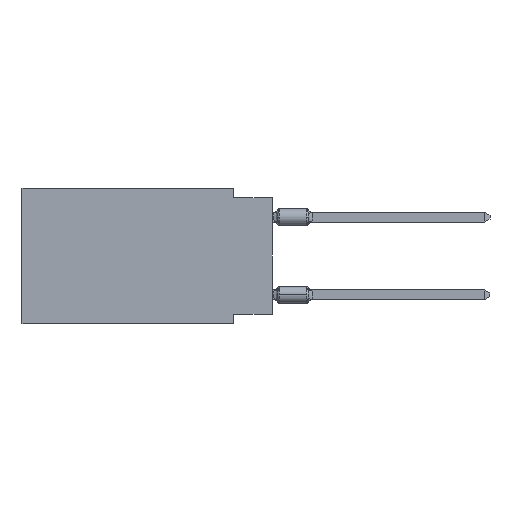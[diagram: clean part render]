
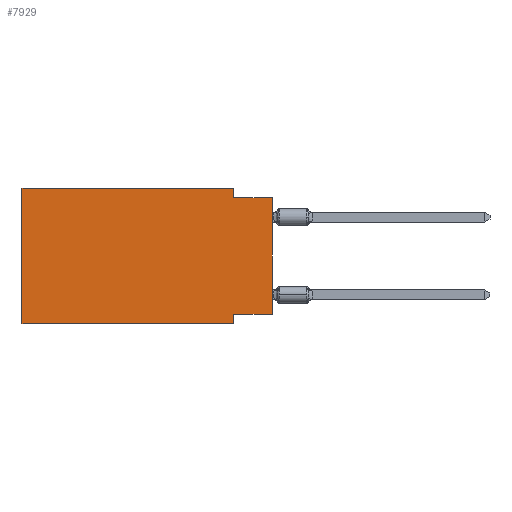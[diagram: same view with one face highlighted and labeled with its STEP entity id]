
A CAD part, left-side view. The second image highlights one B-rep face of the part: STEP entity #7929.
In plain terms, the highlighted planar face has unit normal (-1, 0, 0).
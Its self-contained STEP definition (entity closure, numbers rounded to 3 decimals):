
#190 = CARTESIAN_POINT ( 'NONE',  ( 0., 16.383, -8.89 ) ) ;
#228 = VECTOR ( 'NONE', #21520, 1000. ) ;
#433 = LINE ( 'NONE', #3594, #9265 ) ;
#537 = CARTESIAN_POINT ( 'NONE',  ( 0., 2.54, -8.89 ) ) ;
#577 = LINE ( 'NONE', #10578, #9634 ) ;
#954 = CARTESIAN_POINT ( 'NONE',  ( 0., 2.54, -8.255 ) ) ;
#1461 = PLANE ( 'NONE',  #11725 ) ;
#1567 = DIRECTION ( 'NONE',  ( 1., 0., 0. ) ) ;
#1954 = LINE ( 'NONE', #16637, #19149 ) ;
#2015 = CARTESIAN_POINT ( 'NONE',  ( 0., 2.54, -0.635 ) ) ;
#2173 = CARTESIAN_POINT ( 'NONE',  ( 0., 0., -0.635 ) ) ;
#2688 = VECTOR ( 'NONE', #8791, 1000. ) ;
#3594 = CARTESIAN_POINT ( 'NONE',  ( 0., 16.383, 0. ) ) ;
#4044 = VECTOR ( 'NONE', #10861, 1000. ) ;
#4230 = LINE ( 'NONE', #537, #4044 ) ;
#4486 = CARTESIAN_POINT ( 'NONE',  ( 0., 2.54, 0. ) ) ;
#4720 = DIRECTION ( 'NONE',  ( 0., 0., -1. ) ) ;
#4979 = VERTEX_POINT ( 'NONE', #13889 ) ;
#5195 = ORIENTED_EDGE ( 'NONE', *, *, #10263, .T. ) ;
#5732 = DIRECTION ( 'NONE',  ( 0., 0., 1. ) ) ;
#6154 = EDGE_CURVE ( 'NONE', #19592, #17253, #16729, .T. ) ;
#6299 = CARTESIAN_POINT ( 'NONE',  ( 0., 0., -0.635 ) ) ;
#7164 = DIRECTION ( 'NONE',  ( 0., 0., 1. ) ) ;
#7816 = ORIENTED_EDGE ( 'NONE', *, *, #14226, .F. ) ;
#7929 = ADVANCED_FACE ( 'NONE', ( #13870 ), #1461, .F. ) ;
#8134 = EDGE_CURVE ( 'NONE', #4979, #17988, #577, .T. ) ;
#8254 = CARTESIAN_POINT ( 'NONE',  ( 0., 0., -8.255 ) ) ;
#8571 = DIRECTION ( 'NONE',  ( 0., 1., 0. ) ) ;
#8698 = ORIENTED_EDGE ( 'NONE', *, *, #9793, .F. ) ;
#8791 = DIRECTION ( 'NONE',  ( 0., -1., 0. ) ) ;
#9265 = VECTOR ( 'NONE', #7164, 1000. ) ;
#9379 = CARTESIAN_POINT ( 'NONE',  ( 0., 2.54, -8.89 ) ) ;
#9634 = VECTOR ( 'NONE', #17216, 1000. ) ;
#9793 = EDGE_CURVE ( 'NONE', #17988, #21212, #14392, .T. ) ;
#10032 = EDGE_CURVE ( 'NONE', #10517, #12169, #4230, .T. ) ;
#10263 = EDGE_CURVE ( 'NONE', #16276, #12169, #15208, .T. ) ;
#10517 = VERTEX_POINT ( 'NONE', #954 ) ;
#10578 = CARTESIAN_POINT ( 'NONE',  ( 0., 16.383, 0. ) ) ;
#10861 = DIRECTION ( 'NONE',  ( 0., 0., -1. ) ) ;
#11725 = AXIS2_PLACEMENT_3D ( 'NONE', #13202, #1567, #4720 ) ;
#12169 = VERTEX_POINT ( 'NONE', #9379 ) ;
#12551 = ORIENTED_EDGE ( 'NONE', *, *, #10032, .F. ) ;
#12606 = EDGE_LOOP ( 'NONE', ( #18699, #18980, #8698, #20042, #7816, #5195, #12551, #20224 ) ) ;
#12758 = CARTESIAN_POINT ( 'NONE',  ( 0., 2.54, 0. ) ) ;
#13202 = CARTESIAN_POINT ( 'NONE',  ( 0., 16.383, 0. ) ) ;
#13870 = FACE_OUTER_BOUND ( 'NONE', #12606, .T. ) ;
#13889 = CARTESIAN_POINT ( 'NONE',  ( 0., 16.383, 0. ) ) ;
#14226 = EDGE_CURVE ( 'NONE', #16276, #4979, #433, .T. ) ;
#14262 = EDGE_CURVE ( 'NONE', #21212, #17253, #17069, .T. ) ;
#14324 = VECTOR ( 'NONE', #19393, 1000. ) ;
#14392 = LINE ( 'NONE', #12758, #14324 ) ;
#15208 = LINE ( 'NONE', #190, #228 ) ;
#16276 = VERTEX_POINT ( 'NONE', #16810 ) ;
#16637 = CARTESIAN_POINT ( 'NONE',  ( 0., 0., -8.255 ) ) ;
#16729 = LINE ( 'NONE', #20862, #17120 ) ;
#16810 = CARTESIAN_POINT ( 'NONE',  ( 0., 16.383, -8.89 ) ) ;
#17069 = LINE ( 'NONE', #2173, #2688 ) ;
#17120 = VECTOR ( 'NONE', #5732, 1000. ) ;
#17216 = DIRECTION ( 'NONE',  ( 0., -1., 0. ) ) ;
#17253 = VERTEX_POINT ( 'NONE', #6299 ) ;
#17370 = EDGE_CURVE ( 'NONE', #19592, #10517, #1954, .T. ) ;
#17988 = VERTEX_POINT ( 'NONE', #4486 ) ;
#18699 = ORIENTED_EDGE ( 'NONE', *, *, #6154, .T. ) ;
#18980 = ORIENTED_EDGE ( 'NONE', *, *, #14262, .F. ) ;
#19149 = VECTOR ( 'NONE', #8571, 1000. ) ;
#19393 = DIRECTION ( 'NONE',  ( 0., 0., -1. ) ) ;
#19592 = VERTEX_POINT ( 'NONE', #8254 ) ;
#20042 = ORIENTED_EDGE ( 'NONE', *, *, #8134, .F. ) ;
#20224 = ORIENTED_EDGE ( 'NONE', *, *, #17370, .F. ) ;
#20862 = CARTESIAN_POINT ( 'NONE',  ( 0., 0., 0. ) ) ;
#21212 = VERTEX_POINT ( 'NONE', #2015 ) ;
#21520 = DIRECTION ( 'NONE',  ( 0., -1., 0. ) ) ;
